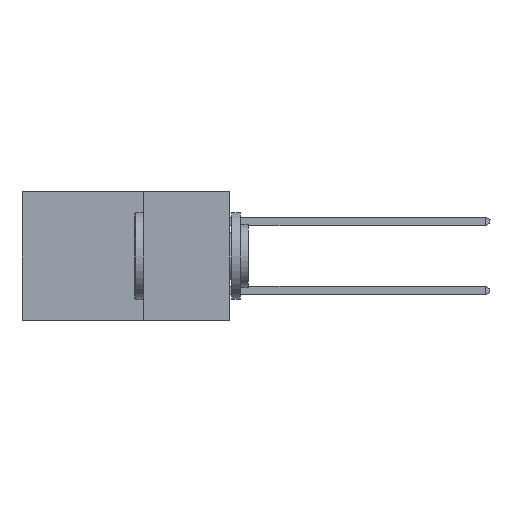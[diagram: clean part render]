
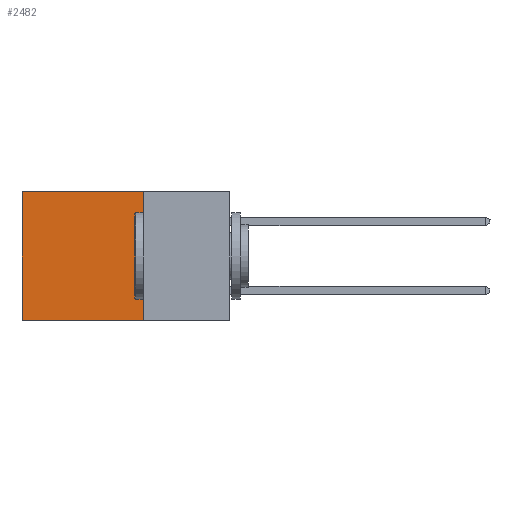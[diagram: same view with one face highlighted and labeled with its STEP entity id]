
A CAD part, left-side view. The second image highlights one B-rep face of the part: STEP entity #2482.
In plain terms, the highlighted planar face has unit normal (-1, 0, 0).
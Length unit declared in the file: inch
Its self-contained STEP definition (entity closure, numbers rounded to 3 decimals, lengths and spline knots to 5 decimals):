
#280 = VECTOR ( 'NONE', #4806, 39.37008 ) ;
#955 = LINE ( 'NONE', #6665, #280 ) ;
#994 = CARTESIAN_POINT ( 'NONE',  ( 0.2615, 0.25, 0. ) ) ;
#1087 = DIRECTION ( 'NONE',  ( 0., 0., -1. ) ) ;
#1630 = CARTESIAN_POINT ( 'NONE',  ( 0.2615, 0.6, -0.37 ) ) ;
#2482 = ADVANCED_FACE ( 'NONE', ( #10673 ), #4931, .F. ) ;
#2499 = DIRECTION ( 'NONE',  ( 0., 0., -1. ) ) ;
#3027 = ORIENTED_EDGE ( 'NONE', *, *, #6823, .F. ) ;
#4806 = DIRECTION ( 'NONE',  ( 0., 1., 0. ) ) ;
#4931 = PLANE ( 'NONE',  #6735 ) ;
#5310 = EDGE_LOOP ( 'NONE', ( #6740, #9517, #3027, #7298 ) ) ;
#5385 = VECTOR ( 'NONE', #5986, 39.37008 ) ;
#5589 = VECTOR ( 'NONE', #11407, 39.37008 ) ;
#5986 = DIRECTION ( 'NONE',  ( 0., 1., 0. ) ) ;
#6029 = VERTEX_POINT ( 'NONE', #11558 ) ;
#6041 = VERTEX_POINT ( 'NONE', #10703 ) ;
#6304 = EDGE_CURVE ( 'NONE', #6029, #8770, #12243, .T. ) ;
#6665 = CARTESIAN_POINT ( 'NONE',  ( 0.2615, 0.25, -0.37 ) ) ;
#6735 = AXIS2_PLACEMENT_3D ( 'NONE', #9707, #7915, #1087 ) ;
#6740 = ORIENTED_EDGE ( 'NONE', *, *, #6304, .T. ) ;
#6823 = EDGE_CURVE ( 'NONE', #12011, #6041, #10160, .T. ) ;
#6929 = EDGE_CURVE ( 'NONE', #6041, #8770, #955, .T. ) ;
#7298 = ORIENTED_EDGE ( 'NONE', *, *, #9096, .T. ) ;
#7915 = DIRECTION ( 'NONE',  ( 1., 0., 0. ) ) ;
#7947 = LINE ( 'NONE', #994, #5385 ) ;
#8770 = VERTEX_POINT ( 'NONE', #12000 ) ;
#9096 = EDGE_CURVE ( 'NONE', #12011, #6029, #7947, .T. ) ;
#9207 = CARTESIAN_POINT ( 'NONE',  ( 0.2615, 0.25, -0.37 ) ) ;
#9517 = ORIENTED_EDGE ( 'NONE', *, *, #6929, .F. ) ;
#9707 = CARTESIAN_POINT ( 'NONE',  ( 0.2615, 0.25, -0.37 ) ) ;
#10160 = LINE ( 'NONE', #9207, #10275 ) ;
#10275 = VECTOR ( 'NONE', #2499, 39.37008 ) ;
#10622 = CARTESIAN_POINT ( 'NONE',  ( 0.2615, 0.25, 0. ) ) ;
#10673 = FACE_OUTER_BOUND ( 'NONE', #5310, .T. ) ;
#10703 = CARTESIAN_POINT ( 'NONE',  ( 0.2615, 0.25, -0.37 ) ) ;
#11407 = DIRECTION ( 'NONE',  ( 0., 0., -1. ) ) ;
#11558 = CARTESIAN_POINT ( 'NONE',  ( 0.2615, 0.6, 0. ) ) ;
#12000 = CARTESIAN_POINT ( 'NONE',  ( 0.2615, 0.6, -0.37 ) ) ;
#12011 = VERTEX_POINT ( 'NONE', #10622 ) ;
#12243 = LINE ( 'NONE', #1630, #5589 ) ;
